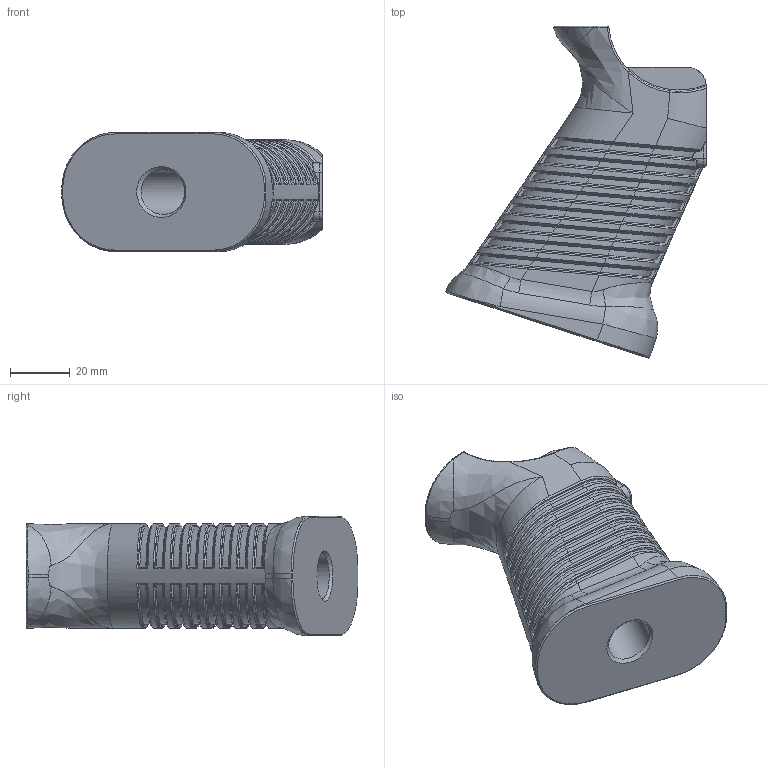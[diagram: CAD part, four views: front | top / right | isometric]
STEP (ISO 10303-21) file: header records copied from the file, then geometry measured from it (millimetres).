
FILE_DESCRIPTION (( 'STEP AP203' ), '1' );
FILE_NAME ('MOD9_pistol_grip.STEP', '2020-06-10T05:00:27', ( '' ), ( '' ), 'SwSTEP 2.0', 'SolidWorks 2016', '' );
FILE_SCHEMA (( 'CONFIG_CONTROL_DESIGN' ));
Products named in the file (1): MOD9_pistol_grip
Bounding box: 87.31 x 111.25 x 40 mm (x, y, z)
Volume: 134075.4 mm3; surface area: 25683.8 mm2
Topology: 1 solids, 1 shells, 634 faces, 1726 edges, 1092 vertices
Faces by surface type: bspline 326, plane 219, cylinder 73, cone 8, torus 8
Full cylindrical faces by diameter (mm): 4.175 x1, 6.605 x1, 15 x1
Entity records: 40533 total; most frequent: CARTESIAN_POINT 26922, ORIENTED_EDGE 3430, DIRECTION 1766, EDGE_CURVE 1715, VERTEX_POINT 1089, VECTOR 894, LINE 894, EDGE_LOOP 642
